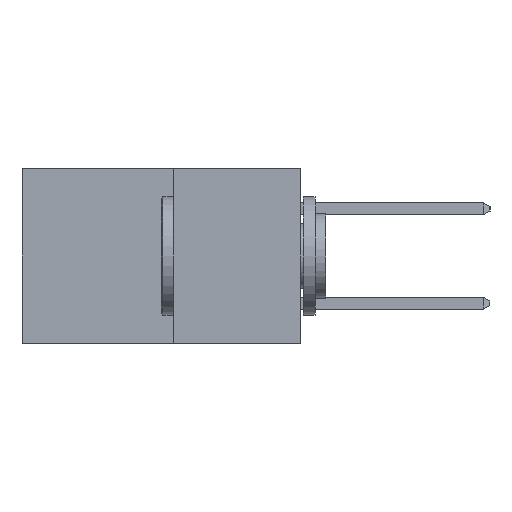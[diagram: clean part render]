
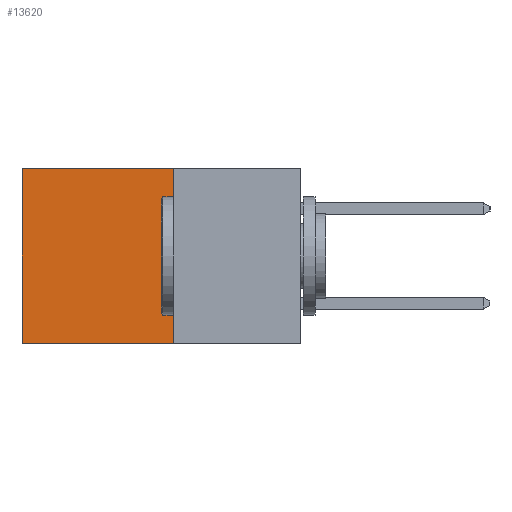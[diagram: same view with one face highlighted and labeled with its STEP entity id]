
A CAD part, left-side view. The second image highlights one B-rep face of the part: STEP entity #13620.
In plain terms, the highlighted planar face has unit normal (-1, 0, 0).
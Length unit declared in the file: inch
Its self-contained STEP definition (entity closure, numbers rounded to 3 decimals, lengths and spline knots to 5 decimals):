
#916 = CARTESIAN_POINT ( 'NONE',  ( 0.277, 0.27, -0.37 ) ) ;
#1227 = VERTEX_POINT ( 'NONE', #5767 ) ;
#1436 = LINE ( 'NONE', #6651, #13129 ) ;
#1663 = LINE ( 'NONE', #12147, #7222 ) ;
#2062 = DIRECTION ( 'NONE',  ( 0., 0., -1. ) ) ;
#2771 = CARTESIAN_POINT ( 'NONE',  ( 0.277, 0.27, -0.37 ) ) ;
#2837 = CARTESIAN_POINT ( 'NONE',  ( 0.277, 0.59, 0. ) ) ;
#2943 = ORIENTED_EDGE ( 'NONE', *, *, #8036, .F. ) ;
#3180 = EDGE_CURVE ( 'NONE', #10554, #1227, #13669, .T. ) ;
#3218 = EDGE_CURVE ( 'NONE', #6280, #6385, #1663, .T. ) ;
#3821 = CARTESIAN_POINT ( 'NONE',  ( 0.277, 0.27, 0. ) ) ;
#4236 = EDGE_LOOP ( 'NONE', ( #4899, #4731, #2943, #5709 ) ) ;
#4731 = ORIENTED_EDGE ( 'NONE', *, *, #3180, .F. ) ;
#4748 = DIRECTION ( 'NONE',  ( 0., 1., 0. ) ) ;
#4883 = CARTESIAN_POINT ( 'NONE',  ( 0.277, 0.27, -0.37 ) ) ;
#4899 = ORIENTED_EDGE ( 'NONE', *, *, #7176, .T. ) ;
#4966 = AXIS2_PLACEMENT_3D ( 'NONE', #916, #8683, #2062 ) ;
#5092 = VECTOR ( 'NONE', #5904, 39.37008 ) ;
#5709 = ORIENTED_EDGE ( 'NONE', *, *, #3218, .T. ) ;
#5767 = CARTESIAN_POINT ( 'NONE',  ( 0.277, 0.59, -0.37 ) ) ;
#5904 = DIRECTION ( 'NONE',  ( 0., 0., -1. ) ) ;
#6280 = VERTEX_POINT ( 'NONE', #3821 ) ;
#6385 = VERTEX_POINT ( 'NONE', #2837 ) ;
#6489 = PLANE ( 'NONE',  #4966 ) ;
#6564 = DIRECTION ( 'NONE',  ( 0., 0., -1. ) ) ;
#6651 = CARTESIAN_POINT ( 'NONE',  ( 0.277, 0.59, -0.37 ) ) ;
#7119 = FACE_OUTER_BOUND ( 'NONE', #4236, .T. ) ;
#7176 = EDGE_CURVE ( 'NONE', #6385, #1227, #1436, .T. ) ;
#7222 = VECTOR ( 'NONE', #7327, 39.37008 ) ;
#7327 = DIRECTION ( 'NONE',  ( 0., 1., 0. ) ) ;
#8001 = LINE ( 'NONE', #4883, #5092 ) ;
#8036 = EDGE_CURVE ( 'NONE', #6280, #10554, #8001, .T. ) ;
#8683 = DIRECTION ( 'NONE',  ( 1., 0., 0. ) ) ;
#8728 = CARTESIAN_POINT ( 'NONE',  ( 0.277, 0.27, -0.37 ) ) ;
#10448 = VECTOR ( 'NONE', #4748, 39.37008 ) ;
#10554 = VERTEX_POINT ( 'NONE', #8728 ) ;
#12147 = CARTESIAN_POINT ( 'NONE',  ( 0.277, 0.27, 0. ) ) ;
#13129 = VECTOR ( 'NONE', #6564, 39.37008 ) ;
#13620 = ADVANCED_FACE ( 'NONE', ( #7119 ), #6489, .F. ) ;
#13669 = LINE ( 'NONE', #2771, #10448 ) ;
